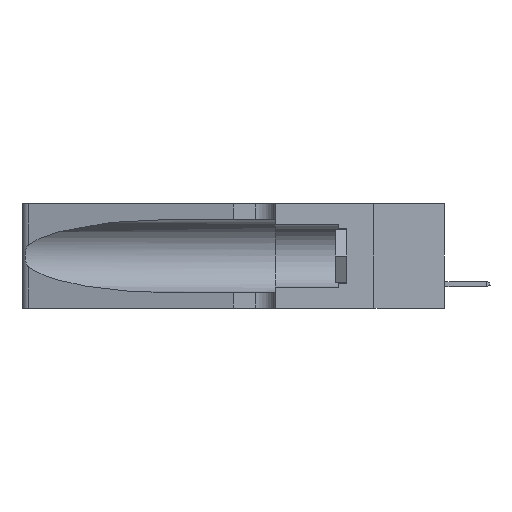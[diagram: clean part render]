
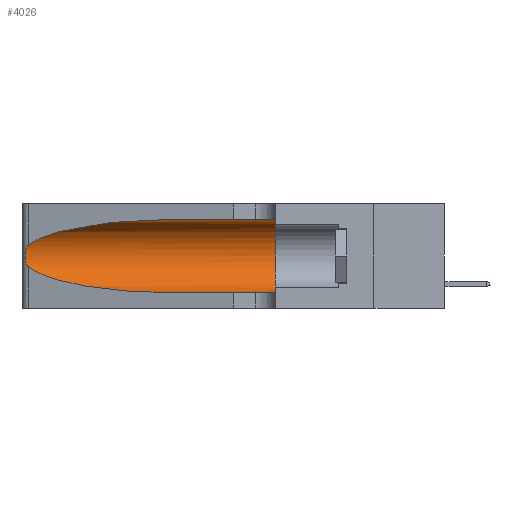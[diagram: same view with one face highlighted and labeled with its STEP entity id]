
A CAD part, left-side view. The second image highlights one B-rep face of the part: STEP entity #4026.
In plain terms, the highlighted cylindrical face has radius 3.308 mm (diameter 6.617 mm), a partial arc.
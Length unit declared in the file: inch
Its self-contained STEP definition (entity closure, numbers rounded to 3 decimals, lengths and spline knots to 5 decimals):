
#175 = ORIENTED_EDGE ( 'NONE', *, *, #30080, .T. ) ;
#576 = CARTESIAN_POINT ( 'NONE',  ( 0.26018, 1.23835, 0.19895 ) ) ;
#601 = ORIENTED_EDGE ( 'NONE', *, *, #12065, .T. ) ;
#1068 = CARTESIAN_POINT ( 'NONE',  ( 0.1305, 0.35, 0.05475 ) ) ;
#1184 = VERTEX_POINT ( 'NONE', #23415 ) ;
#1630 = CARTESIAN_POINT ( 'NONE',  ( 0.25487, 1.22718, 0.14631 ) ) ;
#2732 = ORIENTED_EDGE ( 'NONE', *, *, #10905, .T. ) ;
#3348 = CARTESIAN_POINT ( 'NONE',  ( 0.25487, 1.22718, 0.14631 ) ) ;
#3477 = DIRECTION ( 'NONE',  ( 0., 0., -1. ) ) ;
#4026 = ADVANCED_FACE ( 'NONE', ( #7392 ), #12426, .F. ) ;
#4281 = VECTOR ( 'NONE', #12408, 39.37008 ) ;
#5125 = LINE ( 'NONE', #15085, #4281 ) ;
#5775 =( BOUNDED_CURVE ( )  B_SPLINE_CURVE ( 3, ( #27507, #16609, #16975, #11604 ),
 .UNSPECIFIED., .F., .F. ) 
 B_SPLINE_CURVE_WITH_KNOTS ( ( 4, 4 ),
 ( 1.5708, 2.84003 ),
 .UNSPECIFIED. ) 
 CURVE ( )  GEOMETRIC_REPRESENTATION_ITEM ( )  RATIONAL_B_SPLINE_CURVE ( ( 1., 0.87, 0.87, 1. ) ) 
 REPRESENTATION_ITEM ( '' )  );
#6303 = CARTESIAN_POINT ( 'NONE',  ( 0.26075, 1.23896, 0.178 ) ) ;
#6435 = CARTESIAN_POINT ( 'NONE',  ( 0.25639, 1.23184, 0.21858 ) ) ;
#7392 = FACE_OUTER_BOUND ( 'NONE', #23734, .T. ) ;
#8236 = VERTEX_POINT ( 'NONE', #32756 ) ;
#8428 = VERTEX_POINT ( 'NONE', #25098 ) ;
#8641 = CARTESIAN_POINT ( 'NONE',  ( 0.1305, 0.35, 0.31525 ) ) ;
#8773 = CARTESIAN_POINT ( 'NONE',  ( 0.1305, 0.35, 0.185 ) ) ;
#9576 = ORIENTED_EDGE ( 'NONE', *, *, #12375, .T. ) ;
#10862 = DIRECTION ( 'NONE',  ( 0., -1., 0. ) ) ;
#10905 = EDGE_CURVE ( 'NONE', #26639, #21683, #19891, .T. ) ;
#11475 = CARTESIAN_POINT ( 'NONE',  ( 0.25487, 1.22718, 0.22369 ) ) ;
#11604 = CARTESIAN_POINT ( 'NONE',  ( 0.25487, 1.22718, 0.22369 ) ) ;
#12065 = EDGE_CURVE ( 'NONE', #8428, #1184, #5775, .T. ) ;
#12076 = CARTESIAN_POINT ( 'NONE',  ( 0.1305, 0.72297, 0.05475 ) ) ;
#12375 = EDGE_CURVE ( 'NONE', #8236, #26639, #18659, .T. ) ;
#12408 = DIRECTION ( 'NONE',  ( 0., -1., 0. ) ) ;
#12426 = CYLINDRICAL_SURFACE ( 'NONE', #29193, 0.13025 ) ;
#12794 = CARTESIAN_POINT ( 'NONE',  ( 0.1305, 0.72297, 0.05475 ) ) ;
#12901 = CARTESIAN_POINT ( 'NONE',  ( 0.2373, 1.15595, 0.08982 ) ) ;
#13521 = CIRCLE ( 'NONE', #25132, 0.13025 ) ;
#13831 = DIRECTION ( 'NONE',  ( 0., 0., 1. ) ) ;
#14050 = CARTESIAN_POINT ( 'NONE',  ( 0.25555, 1.22993, 0.14849 ) ) ;
#14053 = CARTESIAN_POINT ( 'NONE',  ( 0.1305, 1.61858, 0.185 ) ) ;
#14172 = B_SPLINE_CURVE_WITH_KNOTS ( 'NONE', 3,
 ( #11475, #14288, #6435, #27629, #29945, #576, #19245, #6303, #22384, #32494, #16843, #19485, #14050, #3348 ),
 .UNSPECIFIED., .F., .F.,
 ( 4, 2, 2, 2, 2, 2, 4 ),
 ( 0., 0.00027, 0.00053, 0.00107, 0.0016, 0.00187, 0.00214 ),
 .UNSPECIFIED. ) ;
#14288 = CARTESIAN_POINT ( 'NONE',  ( 0.25555, 1.22994, 0.2215 ) ) ;
#15085 = CARTESIAN_POINT ( 'NONE',  ( 0.1305, 1.61858, 0.31525 ) ) ;
#16609 = CARTESIAN_POINT ( 'NONE',  ( 0.18966, 0.96281, 0.31525 ) ) ;
#16843 = CARTESIAN_POINT ( 'NONE',  ( 0.25789, 1.23486, 0.15765 ) ) ;
#16975 = CARTESIAN_POINT ( 'NONE',  ( 0.2373, 1.15595, 0.28018 ) ) ;
#18659 =( BOUNDED_CURVE ( )  B_SPLINE_CURVE ( 3, ( #1630, #12901, #28791, #12794 ),
 .UNSPECIFIED., .F., .F. ) 
 B_SPLINE_CURVE_WITH_KNOTS ( ( 4, 4 ),
 ( 3.44316, 4.71239 ),
 .UNSPECIFIED. ) 
 CURVE ( )  GEOMETRIC_REPRESENTATION_ITEM ( )  RATIONAL_B_SPLINE_CURVE ( ( 1., 0.87, 0.87, 1. ) ) 
 REPRESENTATION_ITEM ( '' )  );
#18666 = VECTOR ( 'NONE', #10862, 39.37008 ) ;
#19245 = CARTESIAN_POINT ( 'NONE',  ( 0.26075, 1.23896, 0.19203 ) ) ;
#19485 = CARTESIAN_POINT ( 'NONE',  ( 0.25639, 1.23186, 0.15144 ) ) ;
#19891 = LINE ( 'NONE', #28665, #18666 ) ;
#21683 = VERTEX_POINT ( 'NONE', #1068 ) ;
#22189 = EDGE_CURVE ( 'NONE', #24204, #21683, #13521, .T. ) ;
#22384 = CARTESIAN_POINT ( 'NONE',  ( 0.26017, 1.23833, 0.17102 ) ) ;
#23415 = CARTESIAN_POINT ( 'NONE',  ( 0.25487, 1.22718, 0.22369 ) ) ;
#23734 = EDGE_LOOP ( 'NONE', ( #601, #175, #9576, #2732, #32326, #27035 ) ) ;
#24204 = VERTEX_POINT ( 'NONE', #8641 ) ;
#25098 = CARTESIAN_POINT ( 'NONE',  ( 0.1305, 0.72297, 0.31525 ) ) ;
#25132 = AXIS2_PLACEMENT_3D ( 'NONE', #8773, #29736, #13831 ) ;
#26639 = VERTEX_POINT ( 'NONE', #12076 ) ;
#27035 = ORIENTED_EDGE ( 'NONE', *, *, #29080, .F. ) ;
#27507 = CARTESIAN_POINT ( 'NONE',  ( 0.1305, 0.72297, 0.31525 ) ) ;
#27629 = CARTESIAN_POINT ( 'NONE',  ( 0.25787, 1.23484, 0.2124 ) ) ;
#28665 = CARTESIAN_POINT ( 'NONE',  ( 0.1305, 1.61858, 0.05475 ) ) ;
#28791 = CARTESIAN_POINT ( 'NONE',  ( 0.18966, 0.96281, 0.05475 ) ) ;
#29080 = EDGE_CURVE ( 'NONE', #8428, #24204, #5125, .T. ) ;
#29193 = AXIS2_PLACEMENT_3D ( 'NONE', #14053, #32956, #3477 ) ;
#29736 = DIRECTION ( 'NONE',  ( 0., 1., 0. ) ) ;
#29945 = CARTESIAN_POINT ( 'NONE',  ( 0.25854, 1.2359, 0.20912 ) ) ;
#30080 = EDGE_CURVE ( 'NONE', #1184, #8236, #14172, .T. ) ;
#32326 = ORIENTED_EDGE ( 'NONE', *, *, #22189, .F. ) ;
#32494 = CARTESIAN_POINT ( 'NONE',  ( 0.25856, 1.23593, 0.16098 ) ) ;
#32756 = CARTESIAN_POINT ( 'NONE',  ( 0.25487, 1.22718, 0.14631 ) ) ;
#32956 = DIRECTION ( 'NONE',  ( 0., -1., 0. ) ) ;
